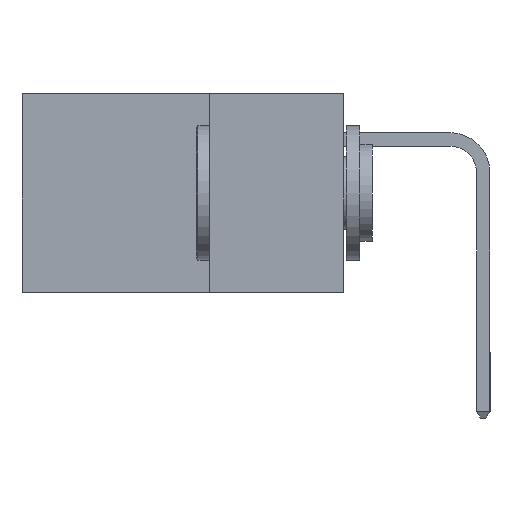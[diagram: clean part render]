
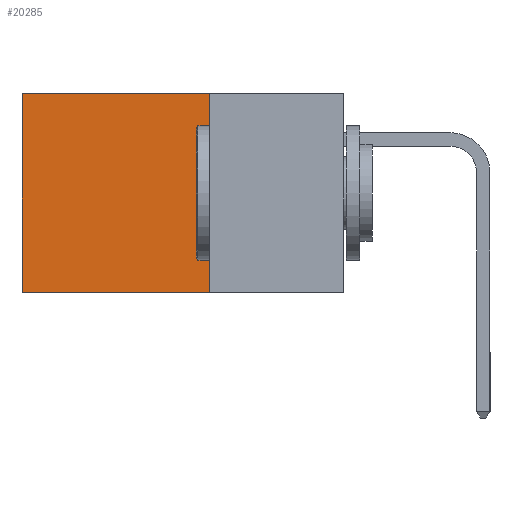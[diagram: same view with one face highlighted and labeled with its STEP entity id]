
A CAD part, left-side view. The second image highlights one B-rep face of the part: STEP entity #20285.
In plain terms, the highlighted planar face has unit normal (-1, 0, 0).
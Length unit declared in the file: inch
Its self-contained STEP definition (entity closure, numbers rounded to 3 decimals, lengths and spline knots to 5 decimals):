
#1296 = LINE ( 'NONE', #13415, #6212 ) ;
#2053 = ORIENTED_EDGE ( 'NONE', *, *, #16451, .T. ) ;
#2541 = EDGE_CURVE ( 'NONE', #24664, #19161, #1296, .T. ) ;
#2770 = CARTESIAN_POINT ( 'NONE',  ( 0.2615, 0.25, 0. ) ) ;
#3588 = DIRECTION ( 'NONE',  ( 0., 1., 0. ) ) ;
#4580 = VECTOR ( 'NONE', #13862, 39.37008 ) ;
#4601 = VECTOR ( 'NONE', #12762, 39.37008 ) ;
#4756 = VECTOR ( 'NONE', #9379, 39.37008 ) ;
#4912 = CARTESIAN_POINT ( 'NONE',  ( 0.2615, 0.25, -0.37 ) ) ;
#5059 = VERTEX_POINT ( 'NONE', #8863 ) ;
#5202 = ORIENTED_EDGE ( 'NONE', *, *, #2541, .T. ) ;
#5453 = DIRECTION ( 'NONE',  ( 1., 0., 0. ) ) ;
#6212 = VECTOR ( 'NONE', #3588, 39.37008 ) ;
#7438 = PLANE ( 'NONE',  #14456 ) ;
#8863 = CARTESIAN_POINT ( 'NONE',  ( 0.2615, 0.6, -0.37 ) ) ;
#8988 = ORIENTED_EDGE ( 'NONE', *, *, #19390, .F. ) ;
#9379 = DIRECTION ( 'NONE',  ( 0., 1., 0. ) ) ;
#10311 = EDGE_LOOP ( 'NONE', ( #2053, #12736, #8988, #5202 ) ) ;
#10312 = VERTEX_POINT ( 'NONE', #12039 ) ;
#12039 = CARTESIAN_POINT ( 'NONE',  ( 0.2615, 0.25, -0.37 ) ) ;
#12736 = ORIENTED_EDGE ( 'NONE', *, *, #25489, .F. ) ;
#12762 = DIRECTION ( 'NONE',  ( 0., 0., -1. ) ) ;
#13415 = CARTESIAN_POINT ( 'NONE',  ( 0.2615, 0.25, 0. ) ) ;
#13612 = CARTESIAN_POINT ( 'NONE',  ( 0.2615, 0.6, 0. ) ) ;
#13862 = DIRECTION ( 'NONE',  ( 0., 0., -1. ) ) ;
#14456 = AXIS2_PLACEMENT_3D ( 'NONE', #23823, #5453, #23959 ) ;
#15893 = LINE ( 'NONE', #19822, #4580 ) ;
#16451 = EDGE_CURVE ( 'NONE', #19161, #5059, #15893, .T. ) ;
#19161 = VERTEX_POINT ( 'NONE', #13612 ) ;
#19390 = EDGE_CURVE ( 'NONE', #24664, #10312, #23254, .T. ) ;
#19777 = LINE ( 'NONE', #23645, #4756 ) ;
#19822 = CARTESIAN_POINT ( 'NONE',  ( 0.2615, 0.6, -0.37 ) ) ;
#20285 = ADVANCED_FACE ( 'NONE', ( #25812 ), #7438, .F. ) ;
#23254 = LINE ( 'NONE', #4912, #4601 ) ;
#23645 = CARTESIAN_POINT ( 'NONE',  ( 0.2615, 0.25, -0.37 ) ) ;
#23823 = CARTESIAN_POINT ( 'NONE',  ( 0.2615, 0.25, -0.37 ) ) ;
#23959 = DIRECTION ( 'NONE',  ( 0., 0., -1. ) ) ;
#24664 = VERTEX_POINT ( 'NONE', #2770 ) ;
#25489 = EDGE_CURVE ( 'NONE', #10312, #5059, #19777, .T. ) ;
#25812 = FACE_OUTER_BOUND ( 'NONE', #10311, .T. ) ;
